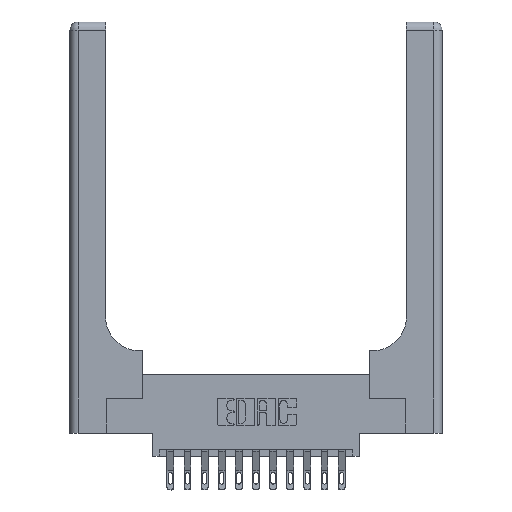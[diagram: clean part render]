
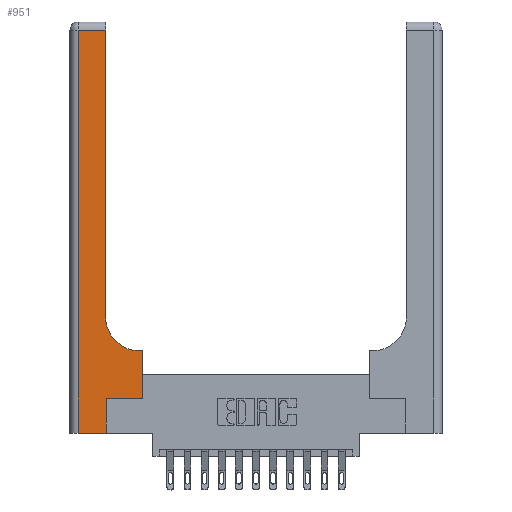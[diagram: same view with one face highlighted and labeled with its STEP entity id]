
A CAD part, top view. The second image highlights one B-rep face of the part: STEP entity #951.
In plain terms, the highlighted planar face has unit normal (0, 0, 1).
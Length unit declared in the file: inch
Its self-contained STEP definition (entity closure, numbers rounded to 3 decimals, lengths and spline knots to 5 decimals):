
#1 = LINE ( 'NONE', #3904, #7392 ) ;
#750 = ORIENTED_EDGE ( 'NONE', *, *, #5059, .T. ) ;
#808 = DIRECTION ( 'NONE',  ( -1., 0., 0. ) ) ;
#951 = ADVANCED_FACE ( 'NONE', ( #3436 ), #14238, .F. ) ;
#1033 = VECTOR ( 'NONE', #5553, 39.37008 ) ;
#1298 = DIRECTION ( 'NONE',  ( 0., 0., -1. ) ) ;
#1449 = LINE ( 'NONE', #12090, #1033 ) ;
#1485 = CARTESIAN_POINT ( 'NONE',  ( 0., 3., 0.37 ) ) ;
#2787 = VERTEX_POINT ( 'NONE', #11513 ) ;
#2814 = ORIENTED_EDGE ( 'NONE', *, *, #11754, .T. ) ;
#2860 = VERTEX_POINT ( 'NONE', #5046 ) ;
#3002 = ORIENTED_EDGE ( 'NONE', *, *, #14650, .T. ) ;
#3134 = VECTOR ( 'NONE', #9771, 39.37008 ) ;
#3436 = FACE_OUTER_BOUND ( 'NONE', #7536, .T. ) ;
#3705 = CIRCLE ( 'NONE', #8983, 0.25 ) ;
#3904 = CARTESIAN_POINT ( 'NONE',  ( 0.26, 3., 0.37 ) ) ;
#3955 = CARTESIAN_POINT ( 'NONE',  ( 0.51, 0.6, 0.37 ) ) ;
#4508 = CARTESIAN_POINT ( 'NONE',  ( 0.528, 0.25, 0.37 ) ) ;
#4643 = DIRECTION ( 'NONE',  ( 1., 0., 0. ) ) ;
#4760 = CARTESIAN_POINT ( 'NONE',  ( 0.06, 0., 0.37 ) ) ;
#4817 = CARTESIAN_POINT ( 'NONE',  ( 0.51, 0.85, 0.37 ) ) ;
#4946 = LINE ( 'NONE', #13767, #11899 ) ;
#4996 = CARTESIAN_POINT ( 'NONE',  ( 0.26, 0.85, 0.37 ) ) ;
#5046 = CARTESIAN_POINT ( 'NONE',  ( 0.265, 0., 0.37 ) ) ;
#5059 = EDGE_CURVE ( 'NONE', #6700, #5511, #5390, .T. ) ;
#5081 = ORIENTED_EDGE ( 'NONE', *, *, #7354, .T. ) ;
#5328 = LINE ( 'NONE', #11980, #11475 ) ;
#5390 = LINE ( 'NONE', #12352, #11940 ) ;
#5511 = VERTEX_POINT ( 'NONE', #15897 ) ;
#5553 = DIRECTION ( 'NONE',  ( 0., -1., 0. ) ) ;
#6128 = DIRECTION ( 'NONE',  ( 1., 0., 0. ) ) ;
#6193 = LINE ( 'NONE', #4508, #3134 ) ;
#6255 = VECTOR ( 'NONE', #4643, 39.37008 ) ;
#6277 = ORIENTED_EDGE ( 'NONE', *, *, #7001, .T. ) ;
#6700 = VERTEX_POINT ( 'NONE', #14479 ) ;
#6754 = CARTESIAN_POINT ( 'NONE',  ( 0.06, 2.94, 0.37 ) ) ;
#7001 = EDGE_CURVE ( 'NONE', #2787, #12909, #5328, .T. ) ;
#7213 = DIRECTION ( 'NONE',  ( 0., 1., 0. ) ) ;
#7248 = EDGE_CURVE ( 'NONE', #2860, #6700, #4946, .T. ) ;
#7354 = EDGE_CURVE ( 'NONE', #9374, #14550, #3705, .T. ) ;
#7392 = VECTOR ( 'NONE', #9094, 39.37008 ) ;
#7484 = EDGE_CURVE ( 'NONE', #12098, #9374, #9006, .T. ) ;
#7536 = EDGE_LOOP ( 'NONE', ( #3002, #6277, #15931, #2814, #14079, #750, #7724, #14732, #5081 ) ) ;
#7657 = CARTESIAN_POINT ( 'NONE',  ( 0.26, 0.6, 0.37 ) ) ;
#7724 = ORIENTED_EDGE ( 'NONE', *, *, #13726, .T. ) ;
#7922 = CARTESIAN_POINT ( 'NONE',  ( 0.528, 0.6, 0.37 ) ) ;
#8983 = AXIS2_PLACEMENT_3D ( 'NONE', #4817, #13988, #6128 ) ;
#9006 = LINE ( 'NONE', #7657, #12111 ) ;
#9094 = DIRECTION ( 'NONE',  ( 0., 1., 0. ) ) ;
#9374 = VERTEX_POINT ( 'NONE', #3955 ) ;
#9746 = LINE ( 'NONE', #16399, #6255 ) ;
#9771 = DIRECTION ( 'NONE',  ( 0., 1., 0. ) ) ;
#11032 = DIRECTION ( 'NONE',  ( 1., 0., 0. ) ) ;
#11475 = VECTOR ( 'NONE', #13294, 39.37008 ) ;
#11513 = CARTESIAN_POINT ( 'NONE',  ( 0.26, 2.94, 0.37 ) ) ;
#11754 = EDGE_CURVE ( 'NONE', #11836, #2860, #9746, .T. ) ;
#11836 = VERTEX_POINT ( 'NONE', #4760 ) ;
#11899 = VECTOR ( 'NONE', #7213, 39.37008 ) ;
#11940 = VECTOR ( 'NONE', #11032, 39.37008 ) ;
#11980 = CARTESIAN_POINT ( 'NONE',  ( 0., 2.94, 0.37 ) ) ;
#12090 = CARTESIAN_POINT ( 'NONE',  ( 0.06, 3., 0.37 ) ) ;
#12098 = VERTEX_POINT ( 'NONE', #7922 ) ;
#12111 = VECTOR ( 'NONE', #12937, 39.37008 ) ;
#12352 = CARTESIAN_POINT ( 'NONE',  ( 0.265, 0.25, 0.37 ) ) ;
#12909 = VERTEX_POINT ( 'NONE', #6754 ) ;
#12937 = DIRECTION ( 'NONE',  ( -1., 0., 0. ) ) ;
#13207 = AXIS2_PLACEMENT_3D ( 'NONE', #1485, #1298, #808 ) ;
#13294 = DIRECTION ( 'NONE',  ( -1., 0., 0. ) ) ;
#13726 = EDGE_CURVE ( 'NONE', #5511, #12098, #6193, .T. ) ;
#13767 = CARTESIAN_POINT ( 'NONE',  ( 0.265, 0., 0.37 ) ) ;
#13988 = DIRECTION ( 'NONE',  ( 0., 0., -1. ) ) ;
#14079 = ORIENTED_EDGE ( 'NONE', *, *, #7248, .T. ) ;
#14238 = PLANE ( 'NONE',  #13207 ) ;
#14479 = CARTESIAN_POINT ( 'NONE',  ( 0.265, 0.25, 0.37 ) ) ;
#14550 = VERTEX_POINT ( 'NONE', #4996 ) ;
#14650 = EDGE_CURVE ( 'NONE', #14550, #2787, #1, .T. ) ;
#14732 = ORIENTED_EDGE ( 'NONE', *, *, #7484, .T. ) ;
#14838 = EDGE_CURVE ( 'NONE', #12909, #11836, #1449, .T. ) ;
#15897 = CARTESIAN_POINT ( 'NONE',  ( 0.528, 0.25, 0.37 ) ) ;
#15931 = ORIENTED_EDGE ( 'NONE', *, *, #14838, .T. ) ;
#16399 = CARTESIAN_POINT ( 'NONE',  ( 0., 0., 0.37 ) ) ;
